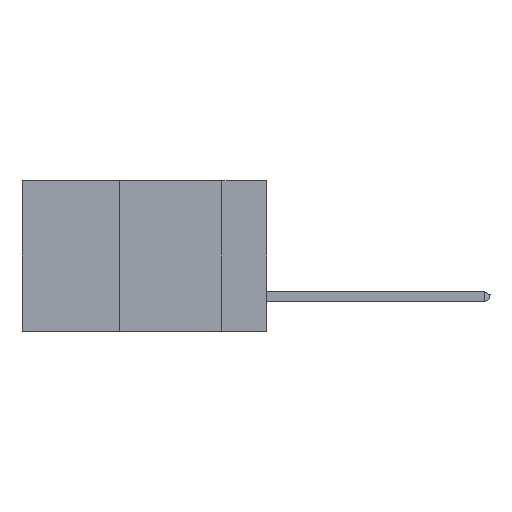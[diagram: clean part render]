
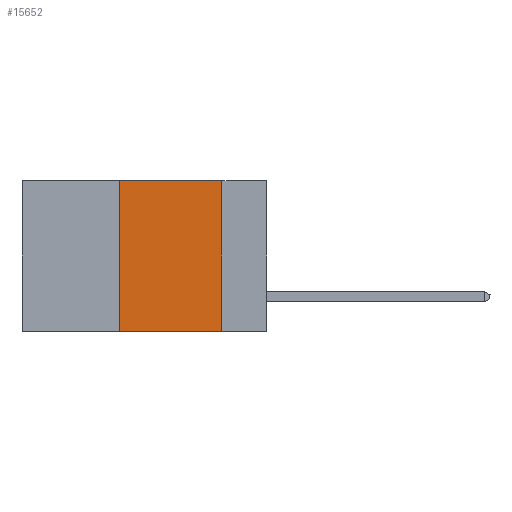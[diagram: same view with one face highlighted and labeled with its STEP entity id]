
A CAD part, left-side view. The second image highlights one B-rep face of the part: STEP entity #15652.
In plain terms, the highlighted planar face has unit normal (-1, 0, 0).
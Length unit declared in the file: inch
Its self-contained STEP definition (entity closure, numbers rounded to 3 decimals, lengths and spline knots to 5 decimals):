
#640 = VERTEX_POINT ( 'NONE', #23580 ) ;
#1223 = ORIENTED_EDGE ( 'NONE', *, *, #20509, .F. ) ;
#2819 = CARTESIAN_POINT ( 'NONE',  ( 0., 0.36, 0. ) ) ;
#2837 = AXIS2_PLACEMENT_3D ( 'NONE', #14383, #14156, #21812 ) ;
#3022 = DIRECTION ( 'NONE',  ( 0., 0., -1. ) ) ;
#3889 = VECTOR ( 'NONE', #12626, 39.37008 ) ;
#4170 = VERTEX_POINT ( 'NONE', #15801 ) ;
#4554 = VERTEX_POINT ( 'NONE', #2819 ) ;
#4971 = LINE ( 'NONE', #14134, #3889 ) ;
#6670 = CARTESIAN_POINT ( 'NONE',  ( 0., 0.11, 0. ) ) ;
#6746 = PLANE ( 'NONE',  #2837 ) ;
#7001 = FACE_OUTER_BOUND ( 'NONE', #17601, .T. ) ;
#7149 = ORIENTED_EDGE ( 'NONE', *, *, #20669, .T. ) ;
#7251 = EDGE_CURVE ( 'NONE', #4170, #4554, #10880, .T. ) ;
#9694 = VECTOR ( 'NONE', #3022, 39.37008 ) ;
#10639 = CARTESIAN_POINT ( 'NONE',  ( 0., 0.36, 0. ) ) ;
#10860 = DIRECTION ( 'NONE',  ( 0., -1., 0. ) ) ;
#10880 = LINE ( 'NONE', #10639, #15631 ) ;
#10948 = CARTESIAN_POINT ( 'NONE',  ( 0., 0.11, 0. ) ) ;
#11517 = VECTOR ( 'NONE', #10860, 39.37008 ) ;
#12626 = DIRECTION ( 'NONE',  ( 0., -1., 0. ) ) ;
#13953 = ORIENTED_EDGE ( 'NONE', *, *, #16592, .F. ) ;
#14134 = CARTESIAN_POINT ( 'NONE',  ( 0., 0.6, 0. ) ) ;
#14156 = DIRECTION ( 'NONE',  ( 1., 0., 0. ) ) ;
#14383 = CARTESIAN_POINT ( 'NONE',  ( 0., 0.6, 0. ) ) ;
#15093 = ORIENTED_EDGE ( 'NONE', *, *, #7251, .F. ) ;
#15226 = CARTESIAN_POINT ( 'NONE',  ( 0., 0.6, -0.37 ) ) ;
#15631 = VECTOR ( 'NONE', #22047, 39.37008 ) ;
#15652 = ADVANCED_FACE ( 'NONE', ( #7001 ), #6746, .F. ) ;
#15801 = CARTESIAN_POINT ( 'NONE',  ( 0., 0.36, -0.37 ) ) ;
#16438 = LINE ( 'NONE', #6670, #9694 ) ;
#16592 = EDGE_CURVE ( 'NONE', #19096, #640, #16438, .T. ) ;
#16879 = LINE ( 'NONE', #15226, #11517 ) ;
#17601 = EDGE_LOOP ( 'NONE', ( #13953, #1223, #15093, #7149 ) ) ;
#19096 = VERTEX_POINT ( 'NONE', #10948 ) ;
#20509 = EDGE_CURVE ( 'NONE', #4554, #19096, #4971, .T. ) ;
#20669 = EDGE_CURVE ( 'NONE', #4170, #640, #16879, .T. ) ;
#21812 = DIRECTION ( 'NONE',  ( 0., 0., -1. ) ) ;
#22047 = DIRECTION ( 'NONE',  ( 0., 0., 1. ) ) ;
#23580 = CARTESIAN_POINT ( 'NONE',  ( 0., 0.11, -0.37 ) ) ;
